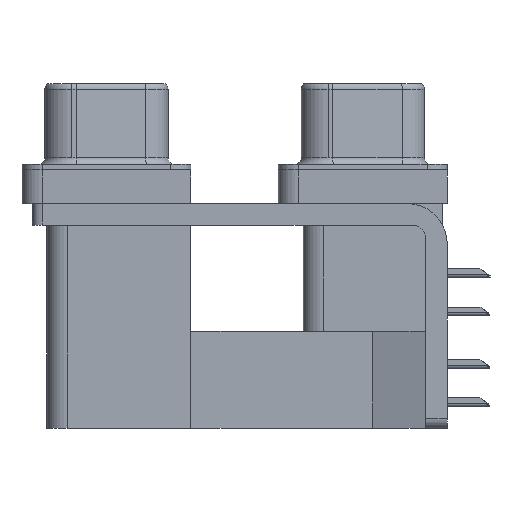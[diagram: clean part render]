
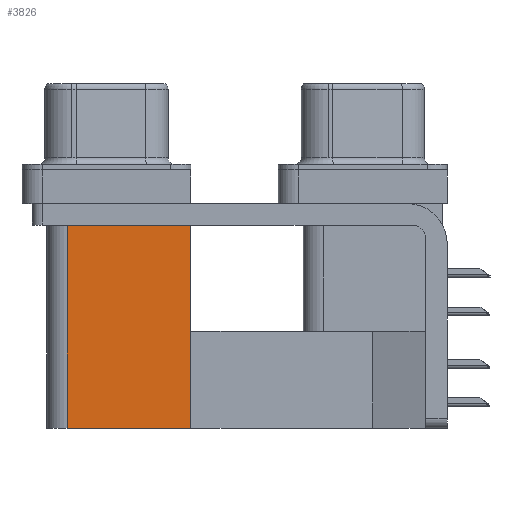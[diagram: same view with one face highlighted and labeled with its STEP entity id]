
A CAD part, left-side view. The second image highlights one B-rep face of the part: STEP entity #3826.
In plain terms, the highlighted planar face has unit normal (-1, 0, 0).
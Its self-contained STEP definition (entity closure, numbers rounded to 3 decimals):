
#1647 = DIRECTION ( 'NONE',  ( 0., 1., 0. ) ) ;
#2615 = VECTOR ( 'NONE', #15105, 1000. ) ;
#3826 = ADVANCED_FACE ( 'NONE', ( #25654 ), #13261, .F. ) ;
#5419 = LINE ( 'NONE', #7112, #14336 ) ;
#5581 = DIRECTION ( 'NONE',  ( 1., 0., 0. ) ) ;
#7112 = CARTESIAN_POINT ( 'NONE',  ( 3.79, 12.775, -19.2 ) ) ;
#7373 = ORIENTED_EDGE ( 'NONE', *, *, #17051, .F. ) ;
#7783 = DIRECTION ( 'NONE',  ( 0., 1., 0. ) ) ;
#7831 = CARTESIAN_POINT ( 'NONE',  ( 3.79, 21.975, -2.5 ) ) ;
#10531 = CARTESIAN_POINT ( 'NONE',  ( 3.79, 21.975, -19.2 ) ) ;
#11172 = ORIENTED_EDGE ( 'NONE', *, *, #24001, .T. ) ;
#11499 = VERTEX_POINT ( 'NONE', #10531 ) ;
#13261 = PLANE ( 'NONE',  #18526 ) ;
#13407 = VECTOR ( 'NONE', #13451, 1000. ) ;
#13451 = DIRECTION ( 'NONE',  ( 0., 0., 1. ) ) ;
#14336 = VECTOR ( 'NONE', #1647, 1000. ) ;
#14725 = LINE ( 'NONE', #22696, #23418 ) ;
#14826 = ORIENTED_EDGE ( 'NONE', *, *, #23541, .F. ) ;
#15105 = DIRECTION ( 'NONE',  ( 0., 1., 0. ) ) ;
#15373 = CARTESIAN_POINT ( 'NONE',  ( 3.79, 12.775, -2.5 ) ) ;
#15404 = LINE ( 'NONE', #19459, #13407 ) ;
#16171 = DIRECTION ( 'NONE',  ( 0., 0., 1. ) ) ;
#16275 = ORIENTED_EDGE ( 'NONE', *, *, #23872, .T. ) ;
#17051 = EDGE_CURVE ( 'NONE', #23382, #11499, #5419, .T. ) ;
#18526 = AXIS2_PLACEMENT_3D ( 'NONE', #21233, #5581, #7783 ) ;
#18678 = CARTESIAN_POINT ( 'NONE',  ( 3.79, 12.775, -19.2 ) ) ;
#19104 = CARTESIAN_POINT ( 'NONE',  ( 3.79, 12.775, -2.5 ) ) ;
#19459 = CARTESIAN_POINT ( 'NONE',  ( 3.79, 21.975, -19.2 ) ) ;
#19544 = VERTEX_POINT ( 'NONE', #7831 ) ;
#20848 = LINE ( 'NONE', #15373, #2615 ) ;
#21233 = CARTESIAN_POINT ( 'NONE',  ( 3.79, 12.775, -19.2 ) ) ;
#22308 = EDGE_LOOP ( 'NONE', ( #11172, #14826, #7373, #16275 ) ) ;
#22696 = CARTESIAN_POINT ( 'NONE',  ( 3.79, 12.775, -19.2 ) ) ;
#23382 = VERTEX_POINT ( 'NONE', #18678 ) ;
#23418 = VECTOR ( 'NONE', #16171, 1000. ) ;
#23541 = EDGE_CURVE ( 'NONE', #11499, #19544, #15404, .T. ) ;
#23872 = EDGE_CURVE ( 'NONE', #23382, #24979, #14725, .T. ) ;
#24001 = EDGE_CURVE ( 'NONE', #24979, #19544, #20848, .T. ) ;
#24979 = VERTEX_POINT ( 'NONE', #19104 ) ;
#25654 = FACE_OUTER_BOUND ( 'NONE', #22308, .T. ) ;
